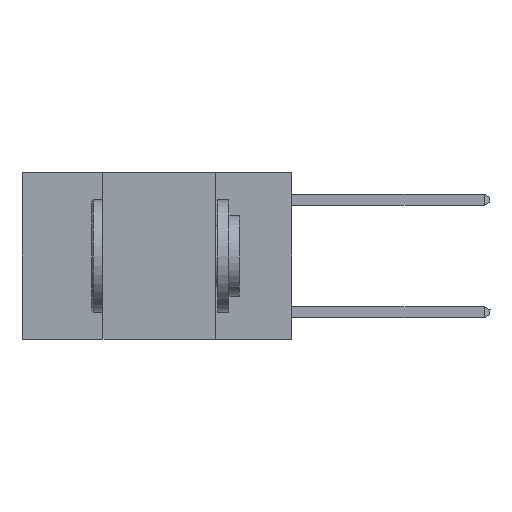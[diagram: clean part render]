
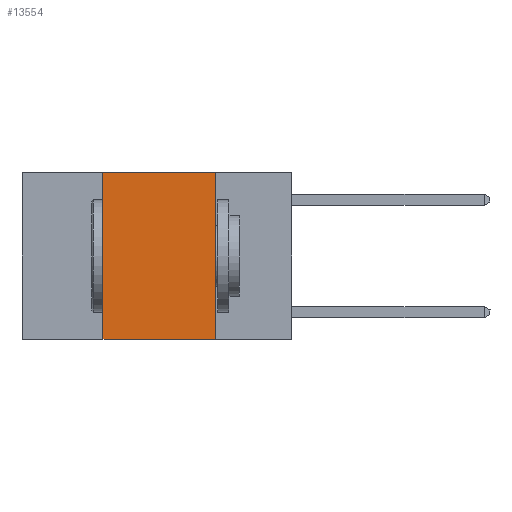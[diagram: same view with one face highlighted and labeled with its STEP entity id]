
A CAD part, left-side view. The second image highlights one B-rep face of the part: STEP entity #13554.
In plain terms, the highlighted planar face has unit normal (-1, 0, 0).
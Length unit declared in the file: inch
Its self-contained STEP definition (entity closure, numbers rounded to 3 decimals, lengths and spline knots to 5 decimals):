
#11 = VECTOR ( 'NONE', #6882, 39.37008 ) ;
#1685 = VERTEX_POINT ( 'NONE', #6416 ) ;
#2118 = EDGE_CURVE ( 'NONE', #1685, #12911, #11484, .T. ) ;
#2217 = DIRECTION ( 'NONE',  ( 1., 0., 0. ) ) ;
#2882 = EDGE_CURVE ( 'NONE', #11759, #8310, #15705, .T. ) ;
#2907 = DIRECTION ( 'NONE',  ( 0., 0., 1. ) ) ;
#3066 = FACE_OUTER_BOUND ( 'NONE', #7622, .T. ) ;
#3376 = EDGE_CURVE ( 'NONE', #12911, #11759, #12093, .T. ) ;
#4037 = DIRECTION ( 'NONE',  ( 0., -1., 0. ) ) ;
#4442 = CARTESIAN_POINT ( 'NONE',  ( 0., 0.17, 0. ) ) ;
#6416 = CARTESIAN_POINT ( 'NONE',  ( 0., 0.42, -0.37 ) ) ;
#6882 = DIRECTION ( 'NONE',  ( 0., -1., 0. ) ) ;
#7455 = ORIENTED_EDGE ( 'NONE', *, *, #2882, .F. ) ;
#7622 = EDGE_LOOP ( 'NONE', ( #7455, #7817, #8248, #8595 ) ) ;
#7738 = VECTOR ( 'NONE', #2907, 39.37008 ) ;
#7779 = CARTESIAN_POINT ( 'NONE',  ( 0., 0.6, 0. ) ) ;
#7817 = ORIENTED_EDGE ( 'NONE', *, *, #3376, .F. ) ;
#7917 = VECTOR ( 'NONE', #14236, 39.37008 ) ;
#8248 = ORIENTED_EDGE ( 'NONE', *, *, #2118, .F. ) ;
#8310 = VERTEX_POINT ( 'NONE', #11467 ) ;
#8459 = VECTOR ( 'NONE', #4037, 39.37008 ) ;
#8517 = CARTESIAN_POINT ( 'NONE',  ( 0., 0.42, 0. ) ) ;
#8595 = ORIENTED_EDGE ( 'NONE', *, *, #16553, .T. ) ;
#10660 = PLANE ( 'NONE',  #15113 ) ;
#11467 = CARTESIAN_POINT ( 'NONE',  ( 0., 0.17, -0.37 ) ) ;
#11484 = LINE ( 'NONE', #8517, #7738 ) ;
#11759 = VERTEX_POINT ( 'NONE', #17854 ) ;
#12077 = DIRECTION ( 'NONE',  ( 0., 0., -1. ) ) ;
#12093 = LINE ( 'NONE', #16500, #11 ) ;
#12212 = LINE ( 'NONE', #13821, #8459 ) ;
#12911 = VERTEX_POINT ( 'NONE', #14838 ) ;
#13554 = ADVANCED_FACE ( 'NONE', ( #3066 ), #10660, .F. ) ;
#13821 = CARTESIAN_POINT ( 'NONE',  ( 0., 0.6, -0.37 ) ) ;
#14236 = DIRECTION ( 'NONE',  ( 0., 0., -1. ) ) ;
#14838 = CARTESIAN_POINT ( 'NONE',  ( 0., 0.42, 0. ) ) ;
#15113 = AXIS2_PLACEMENT_3D ( 'NONE', #7779, #2217, #12077 ) ;
#15705 = LINE ( 'NONE', #4442, #7917 ) ;
#16500 = CARTESIAN_POINT ( 'NONE',  ( 0., 0.6, 0. ) ) ;
#16553 = EDGE_CURVE ( 'NONE', #1685, #8310, #12212, .T. ) ;
#17854 = CARTESIAN_POINT ( 'NONE',  ( 0., 0.17, 0. ) ) ;
